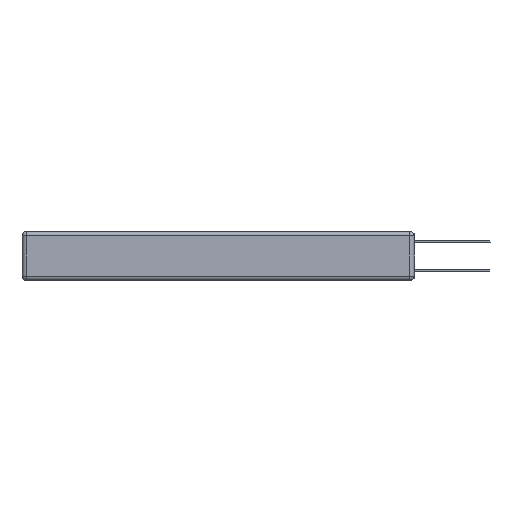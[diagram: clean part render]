
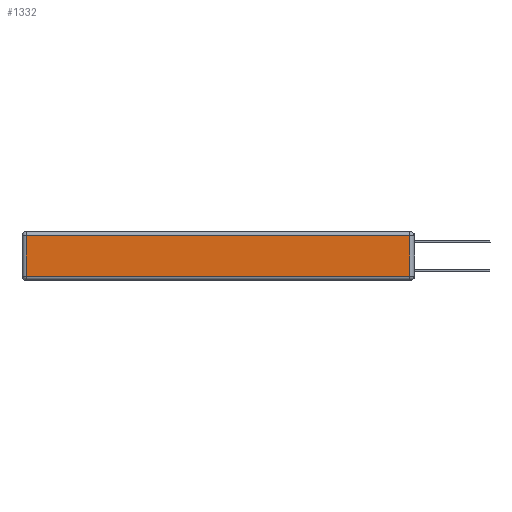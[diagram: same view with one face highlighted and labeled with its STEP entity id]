
A CAD part, left-side view. The second image highlights one B-rep face of the part: STEP entity #1332.
In plain terms, the highlighted planar face has unit normal (-1, 0, 0).
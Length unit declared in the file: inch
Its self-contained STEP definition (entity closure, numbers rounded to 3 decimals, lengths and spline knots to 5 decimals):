
#56 = LINE ( 'NONE', #6190, #8228 ) ;
#417 = ORIENTED_EDGE ( 'NONE', *, *, #10052, .T. ) ;
#447 = VECTOR ( 'NONE', #3946, 39.37008 ) ;
#1332 = ADVANCED_FACE ( 'NONE', ( #4345 ), #3341, .T. ) ;
#1803 = LINE ( 'NONE', #2999, #8439 ) ;
#2073 = CARTESIAN_POINT ( 'NONE',  ( 0., 0., -0.343 ) ) ;
#2220 = VECTOR ( 'NONE', #13159, 39.37008 ) ;
#2999 = CARTESIAN_POINT ( 'NONE',  ( 0., 2.75, -0.03 ) ) ;
#3006 = ORIENTED_EDGE ( 'NONE', *, *, #5070, .T. ) ;
#3341 = PLANE ( 'NONE',  #9845 ) ;
#3479 = VERTEX_POINT ( 'NONE', #5306 ) ;
#3946 = DIRECTION ( 'NONE',  ( 0., -1., 0. ) ) ;
#4345 = FACE_OUTER_BOUND ( 'NONE', #10799, .T. ) ;
#4686 = DIRECTION ( 'NONE',  ( 0., 0., -1. ) ) ;
#5070 = EDGE_CURVE ( 'NONE', #10405, #11663, #56, .T. ) ;
#5306 = CARTESIAN_POINT ( 'NONE',  ( 0., 0.03, -0.313 ) ) ;
#6190 = CARTESIAN_POINT ( 'NONE',  ( 0., 2.72, -0.343 ) ) ;
#7248 = LINE ( 'NONE', #12038, #2220 ) ;
#8228 = VECTOR ( 'NONE', #4686, 39.37008 ) ;
#8439 = VECTOR ( 'NONE', #12429, 39.37008 ) ;
#9170 = DIRECTION ( 'NONE',  ( -1., 0., 0. ) ) ;
#9585 = CARTESIAN_POINT ( 'NONE',  ( 0., 0., -0.313 ) ) ;
#9716 = VERTEX_POINT ( 'NONE', #12947 ) ;
#9845 = AXIS2_PLACEMENT_3D ( 'NONE', #2073, #9170, #11603 ) ;
#10052 = EDGE_CURVE ( 'NONE', #9716, #10405, #1803, .T. ) ;
#10324 = CARTESIAN_POINT ( 'NONE',  ( 0., 2.72, -0.313 ) ) ;
#10405 = VERTEX_POINT ( 'NONE', #13843 ) ;
#10612 = LINE ( 'NONE', #9585, #447 ) ;
#10751 = ORIENTED_EDGE ( 'NONE', *, *, #13660, .T. ) ;
#10799 = EDGE_LOOP ( 'NONE', ( #14422, #10751, #417, #3006 ) ) ;
#11603 = DIRECTION ( 'NONE',  ( 0., 0., 1. ) ) ;
#11663 = VERTEX_POINT ( 'NONE', #10324 ) ;
#12038 = CARTESIAN_POINT ( 'NONE',  ( 0., 0.03, -0.343 ) ) ;
#12429 = DIRECTION ( 'NONE',  ( 0., 1., 0. ) ) ;
#12947 = CARTESIAN_POINT ( 'NONE',  ( 0., 0.03, -0.03 ) ) ;
#13159 = DIRECTION ( 'NONE',  ( 0., 0., 1. ) ) ;
#13660 = EDGE_CURVE ( 'NONE', #3479, #9716, #7248, .T. ) ;
#13843 = CARTESIAN_POINT ( 'NONE',  ( 0., 2.72, -0.03 ) ) ;
#14111 = EDGE_CURVE ( 'NONE', #11663, #3479, #10612, .T. ) ;
#14422 = ORIENTED_EDGE ( 'NONE', *, *, #14111, .T. ) ;
